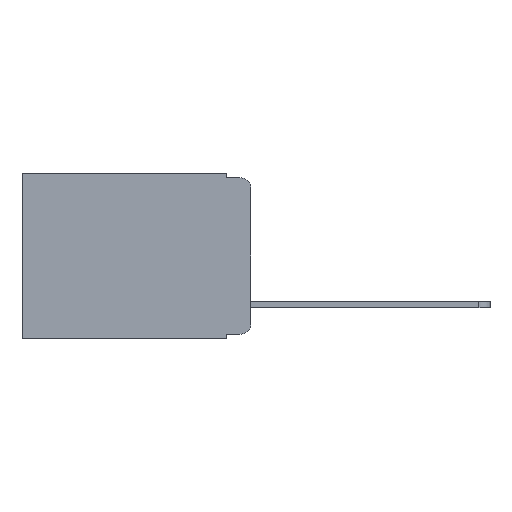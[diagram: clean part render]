
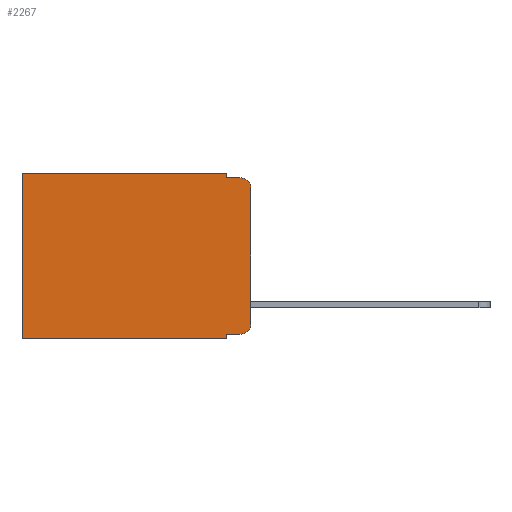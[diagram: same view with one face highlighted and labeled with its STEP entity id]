
A CAD part, left-side view. The second image highlights one B-rep face of the part: STEP entity #2267.
In plain terms, the highlighted planar face has unit normal (-1, 0, 0).
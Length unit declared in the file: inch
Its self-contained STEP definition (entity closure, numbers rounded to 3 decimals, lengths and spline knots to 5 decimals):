
#38 = VECTOR ( 'NONE', #6709, 39.37008 ) ;
#98 = ORIENTED_EDGE ( 'NONE', *, *, #7571, .T. ) ;
#486 = ORIENTED_EDGE ( 'NONE', *, *, #1397, .T. ) ;
#552 = AXIS2_PLACEMENT_3D ( 'NONE', #1502, #5529, #7954 ) ;
#778 = DIRECTION ( 'NONE',  ( 0., 1., 0. ) ) ;
#887 = LINE ( 'NONE', #8261, #10297 ) ;
#1077 = VERTEX_POINT ( 'NONE', #5935 ) ;
#1200 = VERTEX_POINT ( 'NONE', #5266 ) ;
#1337 = CARTESIAN_POINT ( 'NONE',  ( 0.298, 0.051, -0.01 ) ) ;
#1397 = EDGE_CURVE ( 'NONE', #9290, #6137, #5229, .T. ) ;
#1416 = VERTEX_POINT ( 'NONE', #6470 ) ;
#1502 = CARTESIAN_POINT ( 'NONE',  ( 0.298, 0.02, -0.313 ) ) ;
#1663 = DIRECTION ( 'NONE',  ( 0., -1., 0. ) ) ;
#1676 = PLANE ( 'NONE',  #8758 ) ;
#1726 = DIRECTION ( 'NONE',  ( 0., 0., -1. ) ) ;
#1803 = EDGE_CURVE ( 'NONE', #10752, #1416, #5058, .T. ) ;
#1978 = ORIENTED_EDGE ( 'NONE', *, *, #10646, .T. ) ;
#1983 = VECTOR ( 'NONE', #9269, 39.37008 ) ;
#2048 = LINE ( 'NONE', #9529, #9281 ) ;
#2099 = DIRECTION ( 'NONE',  ( 0., 0., -1. ) ) ;
#2168 = EDGE_LOOP ( 'NONE', ( #9166, #8420, #4471, #10674, #1978, #4911, #5105, #8457, #98, #486 ) ) ;
#2249 = CARTESIAN_POINT ( 'NONE',  ( 0.298, 0., -0.313 ) ) ;
#2267 = ADVANCED_FACE ( 'NONE', ( #5048 ), #1676, .F. ) ;
#2268 = LINE ( 'NONE', #3906, #3355 ) ;
#2467 = CARTESIAN_POINT ( 'NONE',  ( 0.298, 0.02, -0.333 ) ) ;
#2468 = EDGE_CURVE ( 'NONE', #10307, #1416, #2268, .T. ) ;
#2675 = CARTESIAN_POINT ( 'NONE',  ( 0.298, 0., -0.03 ) ) ;
#2780 = VECTOR ( 'NONE', #9859, 39.37008 ) ;
#2901 = EDGE_CURVE ( 'NONE', #10417, #1077, #7415, .T. ) ;
#2903 = CARTESIAN_POINT ( 'NONE',  ( 0.298, 0.051, -0.01 ) ) ;
#3021 = DIRECTION ( 'NONE',  ( -1., 0., 0. ) ) ;
#3355 = VECTOR ( 'NONE', #4766, 39.37008 ) ;
#3472 = VECTOR ( 'NONE', #8831, 39.37008 ) ;
#3892 = LINE ( 'NONE', #6348, #2780 ) ;
#3906 = CARTESIAN_POINT ( 'NONE',  ( 0.298, 0.473, 0. ) ) ;
#4012 = EDGE_CURVE ( 'NONE', #7965, #10752, #2048, .T. ) ;
#4227 = EDGE_CURVE ( 'NONE', #10417, #6137, #3892, .T. ) ;
#4258 = CARTESIAN_POINT ( 'NONE',  ( 0.298, 0.051, 0. ) ) ;
#4399 = EDGE_CURVE ( 'NONE', #1200, #5797, #9177, .T. ) ;
#4471 = ORIENTED_EDGE ( 'NONE', *, *, #6934, .F. ) ;
#4753 = DIRECTION ( 'NONE',  ( 0., 0., -1. ) ) ;
#4766 = DIRECTION ( 'NONE',  ( 0., 0., -1. ) ) ;
#4911 = ORIENTED_EDGE ( 'NONE', *, *, #2468, .T. ) ;
#4988 = DIRECTION ( 'NONE',  ( 1., 0., 0. ) ) ;
#5048 = FACE_OUTER_BOUND ( 'NONE', #2168, .T. ) ;
#5058 = LINE ( 'NONE', #6034, #1983 ) ;
#5105 = ORIENTED_EDGE ( 'NONE', *, *, #1803, .F. ) ;
#5229 = CIRCLE ( 'NONE', #552, 0.02 ) ;
#5266 = CARTESIAN_POINT ( 'NONE',  ( 0.298, 0.051, 0. ) ) ;
#5529 = DIRECTION ( 'NONE',  ( -1., 0., 0. ) ) ;
#5797 = VERTEX_POINT ( 'NONE', #2903 ) ;
#5935 = CARTESIAN_POINT ( 'NONE',  ( 0.298, 0.02, -0.01 ) ) ;
#5941 = CARTESIAN_POINT ( 'NONE',  ( 0.298, 0.473, 0. ) ) ;
#5971 = CARTESIAN_POINT ( 'NONE',  ( 0.298, 0.051, -0.343 ) ) ;
#6034 = CARTESIAN_POINT ( 'NONE',  ( 0.298, 0., -0.343 ) ) ;
#6137 = VERTEX_POINT ( 'NONE', #2249 ) ;
#6348 = CARTESIAN_POINT ( 'NONE',  ( 0.298, 0., 0. ) ) ;
#6470 = CARTESIAN_POINT ( 'NONE',  ( 0.298, 0.473, -0.343 ) ) ;
#6642 = CARTESIAN_POINT ( 'NONE',  ( 0.298, 0.051, -0.333 ) ) ;
#6643 = CARTESIAN_POINT ( 'NONE',  ( 0.298, 0.02, -0.03 ) ) ;
#6709 = DIRECTION ( 'NONE',  ( 0., 0., -1. ) ) ;
#6934 = EDGE_CURVE ( 'NONE', #5797, #1077, #8732, .T. ) ;
#7415 = CIRCLE ( 'NONE', #7588, 0.02 ) ;
#7571 = EDGE_CURVE ( 'NONE', #7965, #9290, #8158, .T. ) ;
#7588 = AXIS2_PLACEMENT_3D ( 'NONE', #6643, #3021, #4753 ) ;
#7954 = DIRECTION ( 'NONE',  ( 0., 0., -1. ) ) ;
#7965 = VERTEX_POINT ( 'NONE', #6642 ) ;
#8127 = VECTOR ( 'NONE', #1663, 39.37008 ) ;
#8158 = LINE ( 'NONE', #9037, #8127 ) ;
#8261 = CARTESIAN_POINT ( 'NONE',  ( 0.298, 0., 0. ) ) ;
#8274 = CARTESIAN_POINT ( 'NONE',  ( 0.298, 0., 0. ) ) ;
#8420 = ORIENTED_EDGE ( 'NONE', *, *, #2901, .T. ) ;
#8457 = ORIENTED_EDGE ( 'NONE', *, *, #4012, .F. ) ;
#8732 = LINE ( 'NONE', #1337, #3472 ) ;
#8758 = AXIS2_PLACEMENT_3D ( 'NONE', #8274, #4988, #1726 ) ;
#8831 = DIRECTION ( 'NONE',  ( 0., -1., 0. ) ) ;
#9037 = CARTESIAN_POINT ( 'NONE',  ( 0.298, 0.051, -0.333 ) ) ;
#9166 = ORIENTED_EDGE ( 'NONE', *, *, #4227, .F. ) ;
#9177 = LINE ( 'NONE', #4258, #38 ) ;
#9269 = DIRECTION ( 'NONE',  ( 0., 1., 0. ) ) ;
#9281 = VECTOR ( 'NONE', #2099, 39.37008 ) ;
#9290 = VERTEX_POINT ( 'NONE', #2467 ) ;
#9529 = CARTESIAN_POINT ( 'NONE',  ( 0.298, 0.051, 0. ) ) ;
#9859 = DIRECTION ( 'NONE',  ( 0., 0., -1. ) ) ;
#10297 = VECTOR ( 'NONE', #778, 39.37008 ) ;
#10307 = VERTEX_POINT ( 'NONE', #5941 ) ;
#10417 = VERTEX_POINT ( 'NONE', #2675 ) ;
#10646 = EDGE_CURVE ( 'NONE', #1200, #10307, #887, .T. ) ;
#10674 = ORIENTED_EDGE ( 'NONE', *, *, #4399, .F. ) ;
#10752 = VERTEX_POINT ( 'NONE', #5971 ) ;
